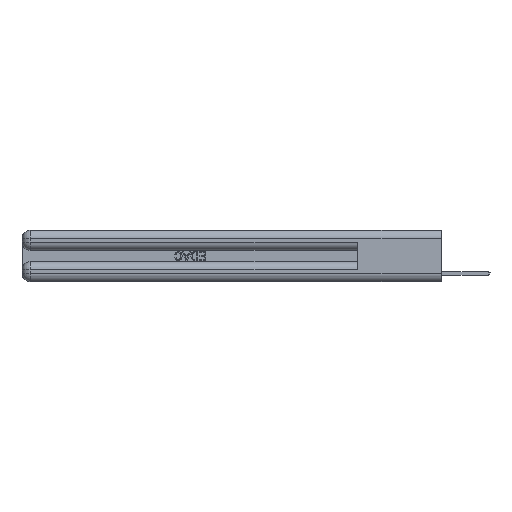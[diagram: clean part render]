
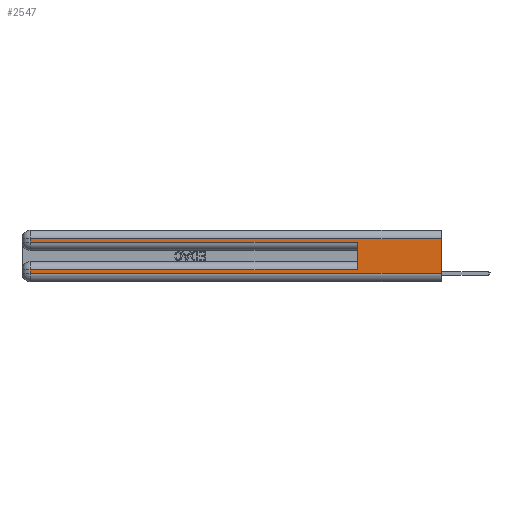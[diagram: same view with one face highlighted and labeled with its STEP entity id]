
A CAD part, left-side view. The second image highlights one B-rep face of the part: STEP entity #2547.
In plain terms, the highlighted planar face has unit normal (-1, 0, 0).
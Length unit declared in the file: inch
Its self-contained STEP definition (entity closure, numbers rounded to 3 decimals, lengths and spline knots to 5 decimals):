
#2028 = CARTESIAN_POINT ( 'NONE',  ( 0., 2.94, 0.06 ) ) ;
#2377 = CARTESIAN_POINT ( 'NONE',  ( 0., 2.94, 0.31 ) ) ;
#2547 = ADVANCED_FACE ( 'NONE', ( #5203 ), #27211, .F. ) ;
#2724 = LINE ( 'NONE', #30002, #24129 ) ;
#3634 = VERTEX_POINT ( 'NONE', #15932 ) ;
#5203 = FACE_OUTER_BOUND ( 'NONE', #24092, .T. ) ;
#5306 = LINE ( 'NONE', #10803, #23187 ) ;
#5506 = AXIS2_PLACEMENT_3D ( 'NONE', #12286, #32208, #11950 ) ;
#5642 = ORIENTED_EDGE ( 'NONE', *, *, #16574, .T. ) ;
#5899 = EDGE_CURVE ( 'NONE', #12717, #26111, #22492, .T. ) ;
#6456 = LINE ( 'NONE', #13025, #29793 ) ;
#6732 = CARTESIAN_POINT ( 'NONE',  ( 0., 0., 0.31 ) ) ;
#6892 = ORIENTED_EDGE ( 'NONE', *, *, #10781, .F. ) ;
#6948 = DIRECTION ( 'NONE',  ( 0., 1., 0. ) ) ;
#7084 = ORIENTED_EDGE ( 'NONE', *, *, #26091, .F. ) ;
#7709 = DIRECTION ( 'NONE',  ( 0., 0., 1. ) ) ;
#7728 = VECTOR ( 'NONE', #6948, 39.37008 ) ;
#7732 = VERTEX_POINT ( 'NONE', #21283 ) ;
#10446 = CARTESIAN_POINT ( 'NONE',  ( 0., 2.94, 0.37 ) ) ;
#10781 = EDGE_CURVE ( 'NONE', #12717, #21478, #6456, .T. ) ;
#10803 = CARTESIAN_POINT ( 'NONE',  ( 0., 0., 0.285 ) ) ;
#11106 = LINE ( 'NONE', #10446, #15020 ) ;
#11305 = ORIENTED_EDGE ( 'NONE', *, *, #17303, .T. ) ;
#11431 = VECTOR ( 'NONE', #28886, 39.37008 ) ;
#11443 = CARTESIAN_POINT ( 'NONE',  ( 0., 0., 0.06 ) ) ;
#11950 = DIRECTION ( 'NONE',  ( 0., 0., -1. ) ) ;
#12110 = ORIENTED_EDGE ( 'NONE', *, *, #5899, .T. ) ;
#12249 = CARTESIAN_POINT ( 'NONE',  ( 0., 2.94, 0.37 ) ) ;
#12286 = CARTESIAN_POINT ( 'NONE',  ( 0., 0., 0.37 ) ) ;
#12717 = VERTEX_POINT ( 'NONE', #21052 ) ;
#12803 = DIRECTION ( 'NONE',  ( 0., 0., -1. ) ) ;
#12873 = VECTOR ( 'NONE', #12803, 39.37008 ) ;
#13025 = CARTESIAN_POINT ( 'NONE',  ( 0., 0., 0.37 ) ) ;
#14308 = CARTESIAN_POINT ( 'NONE',  ( 0., 2.94, 0.085 ) ) ;
#14885 = VERTEX_POINT ( 'NONE', #27864 ) ;
#15020 = VECTOR ( 'NONE', #29820, 39.37008 ) ;
#15932 = CARTESIAN_POINT ( 'NONE',  ( 0., 0.6, 0.285 ) ) ;
#16574 = EDGE_CURVE ( 'NONE', #28583, #21478, #28612, .T. ) ;
#16774 = ORIENTED_EDGE ( 'NONE', *, *, #19563, .T. ) ;
#17303 = EDGE_CURVE ( 'NONE', #7732, #25895, #31270, .T. ) ;
#17525 = DIRECTION ( 'NONE',  ( 0., 1., 0. ) ) ;
#17638 = CARTESIAN_POINT ( 'NONE',  ( 0., 0., 0.085 ) ) ;
#19563 = EDGE_CURVE ( 'NONE', #26111, #14885, #29596, .T. ) ;
#20243 = ORIENTED_EDGE ( 'NONE', *, *, #23279, .T. ) ;
#20285 = CARTESIAN_POINT ( 'NONE',  ( 0., 0., 0.06 ) ) ;
#21052 = CARTESIAN_POINT ( 'NONE',  ( 0., 0., 0.31 ) ) ;
#21283 = CARTESIAN_POINT ( 'NONE',  ( 0., 0.6, 0.085 ) ) ;
#21478 = VERTEX_POINT ( 'NONE', #20285 ) ;
#22076 = EDGE_CURVE ( 'NONE', #25895, #28583, #11106, .T. ) ;
#22492 = LINE ( 'NONE', #6732, #7728 ) ;
#23187 = VECTOR ( 'NONE', #30193, 39.37008 ) ;
#23279 = EDGE_CURVE ( 'NONE', #14885, #3634, #5306, .T. ) ;
#24092 = EDGE_LOOP ( 'NONE', ( #6892, #12110, #16774, #20243, #7084, #11305, #27788, #5642 ) ) ;
#24129 = VECTOR ( 'NONE', #7709, 39.37008 ) ;
#24266 = VECTOR ( 'NONE', #17525, 39.37008 ) ;
#25895 = VERTEX_POINT ( 'NONE', #14308 ) ;
#26091 = EDGE_CURVE ( 'NONE', #7732, #3634, #2724, .T. ) ;
#26111 = VERTEX_POINT ( 'NONE', #2377 ) ;
#27211 = PLANE ( 'NONE',  #5506 ) ;
#27788 = ORIENTED_EDGE ( 'NONE', *, *, #22076, .T. ) ;
#27864 = CARTESIAN_POINT ( 'NONE',  ( 0., 2.94, 0.285 ) ) ;
#28583 = VERTEX_POINT ( 'NONE', #2028 ) ;
#28612 = LINE ( 'NONE', #11443, #11431 ) ;
#28886 = DIRECTION ( 'NONE',  ( 0., -1., 0. ) ) ;
#29596 = LINE ( 'NONE', #12249, #12873 ) ;
#29793 = VECTOR ( 'NONE', #30639, 39.37008 ) ;
#29820 = DIRECTION ( 'NONE',  ( 0., 0., -1. ) ) ;
#30002 = CARTESIAN_POINT ( 'NONE',  ( 0., 0.6, 0.145 ) ) ;
#30193 = DIRECTION ( 'NONE',  ( 0., -1., 0. ) ) ;
#30639 = DIRECTION ( 'NONE',  ( 0., 0., -1. ) ) ;
#31270 = LINE ( 'NONE', #17638, #24266 ) ;
#32208 = DIRECTION ( 'NONE',  ( 1., 0., 0. ) ) ;
